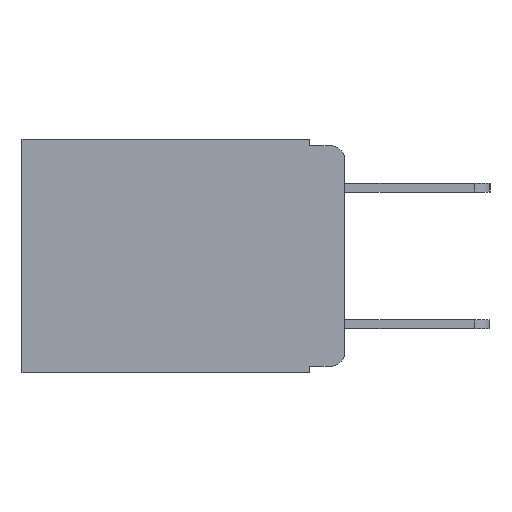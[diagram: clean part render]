
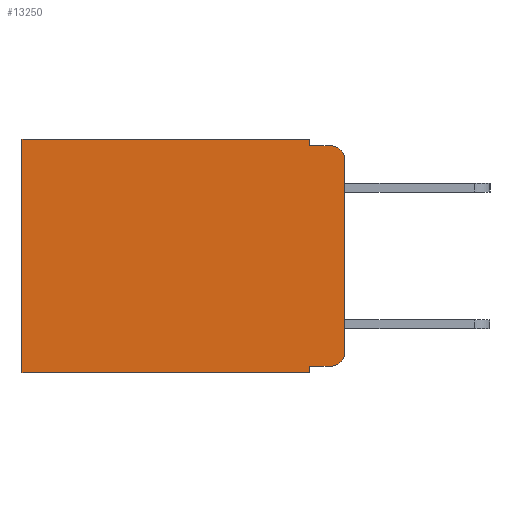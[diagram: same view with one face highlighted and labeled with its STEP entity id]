
A CAD part, left-side view. The second image highlights one B-rep face of the part: STEP entity #13250.
In plain terms, the highlighted planar face has unit normal (-1, 0, 0).
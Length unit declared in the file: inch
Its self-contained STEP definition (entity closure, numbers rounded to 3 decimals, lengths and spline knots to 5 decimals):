
#141 = VERTEX_POINT ( 'NONE', #19125 ) ;
#142 = ORIENTED_EDGE ( 'NONE', *, *, #9118, .F. ) ;
#203 = ORIENTED_EDGE ( 'NONE', *, *, #11402, .F. ) ;
#238 = VECTOR ( 'NONE', #9698, 39.37008 ) ;
#696 = CARTESIAN_POINT ( 'NONE',  ( 0.298, 0.473, 0. ) ) ;
#711 = LINE ( 'NONE', #18350, #20245 ) ;
#1049 = DIRECTION ( 'NONE',  ( 0., 0., -1. ) ) ;
#1152 = ORIENTED_EDGE ( 'NONE', *, *, #14600, .T. ) ;
#1603 = DIRECTION ( 'NONE',  ( 0., 0., -1. ) ) ;
#3307 = PLANE ( 'NONE',  #7109 ) ;
#3885 = VERTEX_POINT ( 'NONE', #10537 ) ;
#4251 = FACE_OUTER_BOUND ( 'NONE', #13330, .T. ) ;
#4306 = VERTEX_POINT ( 'NONE', #13559 ) ;
#4501 = VERTEX_POINT ( 'NONE', #15377 ) ;
#4507 = VECTOR ( 'NONE', #11143, 39.37008 ) ;
#4587 = CARTESIAN_POINT ( 'NONE',  ( 0.298, 0.051, 0. ) ) ;
#4626 = EDGE_CURVE ( 'NONE', #3885, #7810, #13660, .T. ) ;
#4937 = ORIENTED_EDGE ( 'NONE', *, *, #17657, .F. ) ;
#5125 = VECTOR ( 'NONE', #16954, 39.37008 ) ;
#6091 = LINE ( 'NONE', #4587, #238 ) ;
#7109 = AXIS2_PLACEMENT_3D ( 'NONE', #10173, #20742, #11806 ) ;
#7237 = CARTESIAN_POINT ( 'NONE',  ( 0.298, 0.051, 0. ) ) ;
#7637 = CARTESIAN_POINT ( 'NONE',  ( 0.298, 0.051, -0.343 ) ) ;
#7810 = VERTEX_POINT ( 'NONE', #8539 ) ;
#7907 = LINE ( 'NONE', #8463, #16055 ) ;
#8009 = CARTESIAN_POINT ( 'NONE',  ( 0.298, 0., -0.03 ) ) ;
#8184 = VERTEX_POINT ( 'NONE', #8009 ) ;
#8463 = CARTESIAN_POINT ( 'NONE',  ( 0.298, 0.051, -0.333 ) ) ;
#8539 = CARTESIAN_POINT ( 'NONE',  ( 0.298, 0.473, -0.343 ) ) ;
#8720 = DIRECTION ( 'NONE',  ( 0., 1., 0. ) ) ;
#8754 = ORIENTED_EDGE ( 'NONE', *, *, #14812, .T. ) ;
#8821 = LINE ( 'NONE', #13574, #16426 ) ;
#8965 = LINE ( 'NONE', #14360, #4507 ) ;
#9023 = ORIENTED_EDGE ( 'NONE', *, *, #4626, .T. ) ;
#9077 = LINE ( 'NONE', #7237, #5125 ) ;
#9118 = EDGE_CURVE ( 'NONE', #4501, #12030, #9077, .T. ) ;
#9203 = CIRCLE ( 'NONE', #16800, 0.02 ) ;
#9440 = VERTEX_POINT ( 'NONE', #12948 ) ;
#9698 = DIRECTION ( 'NONE',  ( 0., 0., -1. ) ) ;
#9755 = EDGE_CURVE ( 'NONE', #12055, #7810, #711, .T. ) ;
#10038 = VECTOR ( 'NONE', #8720, 39.37008 ) ;
#10118 = DIRECTION ( 'NONE',  ( -1., 0., 0. ) ) ;
#10153 = ORIENTED_EDGE ( 'NONE', *, *, #9755, .F. ) ;
#10173 = CARTESIAN_POINT ( 'NONE',  ( 0.298, 0., 0. ) ) ;
#10219 = DIRECTION ( 'NONE',  ( 0., -1., 0. ) ) ;
#10537 = CARTESIAN_POINT ( 'NONE',  ( 0.298, 0.473, 0. ) ) ;
#10662 = DIRECTION ( 'NONE',  ( 0., 1., 0. ) ) ;
#10896 = ORIENTED_EDGE ( 'NONE', *, *, #17042, .F. ) ;
#11143 = DIRECTION ( 'NONE',  ( 0., 0., -1. ) ) ;
#11213 = CIRCLE ( 'NONE', #15848, 0.02 ) ;
#11388 = ORIENTED_EDGE ( 'NONE', *, *, #13940, .T. ) ;
#11402 = EDGE_CURVE ( 'NONE', #12030, #9440, #8821, .T. ) ;
#11792 = EDGE_CURVE ( 'NONE', #4306, #141, #11213, .T. ) ;
#11806 = DIRECTION ( 'NONE',  ( 0., 0., -1. ) ) ;
#11846 = DIRECTION ( 'NONE',  ( -1., 0., 0. ) ) ;
#12030 = VERTEX_POINT ( 'NONE', #15608 ) ;
#12055 = VERTEX_POINT ( 'NONE', #7637 ) ;
#12077 = ORIENTED_EDGE ( 'NONE', *, *, #11792, .T. ) ;
#12948 = CARTESIAN_POINT ( 'NONE',  ( 0.298, 0.02, -0.01 ) ) ;
#13167 = VECTOR ( 'NONE', #1049, 39.37008 ) ;
#13250 = ADVANCED_FACE ( 'NONE', ( #4251 ), #3307, .F. ) ;
#13330 = EDGE_LOOP ( 'NONE', ( #4937, #1152, #203, #142, #8754, #9023, #10153, #10896, #11388, #12077 ) ) ;
#13559 = CARTESIAN_POINT ( 'NONE',  ( 0.298, 0.02, -0.333 ) ) ;
#13574 = CARTESIAN_POINT ( 'NONE',  ( 0.298, 0.051, -0.01 ) ) ;
#13660 = LINE ( 'NONE', #696, #13167 ) ;
#13940 = EDGE_CURVE ( 'NONE', #19982, #4306, #7907, .T. ) ;
#14360 = CARTESIAN_POINT ( 'NONE',  ( 0.298, 0., 0. ) ) ;
#14600 = EDGE_CURVE ( 'NONE', #8184, #9440, #9203, .T. ) ;
#14803 = LINE ( 'NONE', #19591, #10038 ) ;
#14812 = EDGE_CURVE ( 'NONE', #4501, #3885, #14803, .T. ) ;
#15108 = DIRECTION ( 'NONE',  ( 0., -1., 0. ) ) ;
#15377 = CARTESIAN_POINT ( 'NONE',  ( 0.298, 0.051, 0. ) ) ;
#15608 = CARTESIAN_POINT ( 'NONE',  ( 0.298, 0.051, -0.01 ) ) ;
#15631 = CARTESIAN_POINT ( 'NONE',  ( 0.298, 0.051, -0.333 ) ) ;
#15848 = AXIS2_PLACEMENT_3D ( 'NONE', #20773, #11846, #1603 ) ;
#16055 = VECTOR ( 'NONE', #10219, 39.37008 ) ;
#16426 = VECTOR ( 'NONE', #15108, 39.37008 ) ;
#16800 = AXIS2_PLACEMENT_3D ( 'NONE', #19296, #10118, #20705 ) ;
#16954 = DIRECTION ( 'NONE',  ( 0., 0., -1. ) ) ;
#17042 = EDGE_CURVE ( 'NONE', #19982, #12055, #6091, .T. ) ;
#17657 = EDGE_CURVE ( 'NONE', #8184, #141, #8965, .T. ) ;
#18350 = CARTESIAN_POINT ( 'NONE',  ( 0.298, 0., -0.343 ) ) ;
#19125 = CARTESIAN_POINT ( 'NONE',  ( 0.298, 0., -0.313 ) ) ;
#19296 = CARTESIAN_POINT ( 'NONE',  ( 0.298, 0.02, -0.03 ) ) ;
#19591 = CARTESIAN_POINT ( 'NONE',  ( 0.298, 0., 0. ) ) ;
#19982 = VERTEX_POINT ( 'NONE', #15631 ) ;
#20245 = VECTOR ( 'NONE', #10662, 39.37008 ) ;
#20705 = DIRECTION ( 'NONE',  ( 0., 0., -1. ) ) ;
#20742 = DIRECTION ( 'NONE',  ( 1., 0., 0. ) ) ;
#20773 = CARTESIAN_POINT ( 'NONE',  ( 0.298, 0.02, -0.313 ) ) ;
